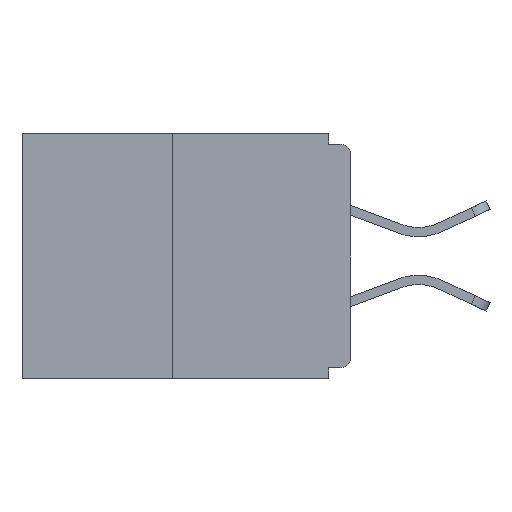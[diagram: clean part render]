
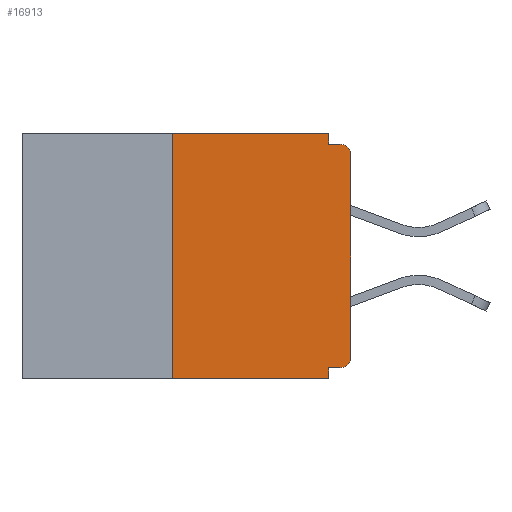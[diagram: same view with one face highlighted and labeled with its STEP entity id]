
A CAD part, left-side view. The second image highlights one B-rep face of the part: STEP entity #16913.
In plain terms, the highlighted planar face has unit normal (-1, 0, 0).
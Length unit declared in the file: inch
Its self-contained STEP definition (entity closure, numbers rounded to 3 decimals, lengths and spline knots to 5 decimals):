
#122 = EDGE_CURVE ( 'NONE', #4354, #20350, #23432, .T. ) ;
#171 = DIRECTION ( 'NONE',  ( 0., 0., -1. ) ) ;
#388 = CARTESIAN_POINT ( 'NONE',  ( 0., 0.015, -0.313 ) ) ;
#556 = ORIENTED_EDGE ( 'NONE', *, *, #22583, .T. ) ;
#1011 = ORIENTED_EDGE ( 'NONE', *, *, #21110, .F. ) ;
#1294 = ORIENTED_EDGE ( 'NONE', *, *, #122, .F. ) ;
#1313 = EDGE_CURVE ( 'NONE', #5069, #13812, #3944, .T. ) ;
#2263 = LINE ( 'NONE', #4719, #18832 ) ;
#3266 = CARTESIAN_POINT ( 'NONE',  ( 0., 0.031, 0. ) ) ;
#3462 = FACE_OUTER_BOUND ( 'NONE', #26568, .T. ) ;
#3801 = EDGE_CURVE ( 'NONE', #5069, #25397, #2263, .T. ) ;
#3944 = CIRCLE ( 'NONE', #6987, 0.015 ) ;
#4184 = EDGE_CURVE ( 'NONE', #10355, #19621, #6949, .T. ) ;
#4192 = VECTOR ( 'NONE', #171, 39.37008 ) ;
#4354 = VERTEX_POINT ( 'NONE', #3266 ) ;
#4472 = DIRECTION ( 'NONE',  ( -1., 0., 0. ) ) ;
#4643 = CARTESIAN_POINT ( 'NONE',  ( 0., 0.25, 0. ) ) ;
#4719 = CARTESIAN_POINT ( 'NONE',  ( 0., 0., -0.328 ) ) ;
#5069 = VERTEX_POINT ( 'NONE', #16992 ) ;
#5516 = DIRECTION ( 'NONE',  ( 0., 0., -1. ) ) ;
#5732 = EDGE_CURVE ( 'NONE', #25242, #19137, #12994, .T. ) ;
#6949 = LINE ( 'NONE', #4643, #9668 ) ;
#6987 = AXIS2_PLACEMENT_3D ( 'NONE', #388, #4472, #17022 ) ;
#7081 = CARTESIAN_POINT ( 'NONE',  ( 0., 0.46, 0. ) ) ;
#7282 = CARTESIAN_POINT ( 'NONE',  ( 0., 0.46, 0. ) ) ;
#7720 = VECTOR ( 'NONE', #17278, 39.37008 ) ;
#8055 = EDGE_CURVE ( 'NONE', #20350, #19137, #13653, .T. ) ;
#8170 = CARTESIAN_POINT ( 'NONE',  ( 0., 0.25, 0. ) ) ;
#8269 = ORIENTED_EDGE ( 'NONE', *, *, #3801, .F. ) ;
#8384 = VECTOR ( 'NONE', #25337, 39.37008 ) ;
#8556 = CARTESIAN_POINT ( 'NONE',  ( 0., 0.031, 0. ) ) ;
#9668 = VECTOR ( 'NONE', #25611, 39.37008 ) ;
#9705 = ORIENTED_EDGE ( 'NONE', *, *, #5732, .T. ) ;
#10355 = VERTEX_POINT ( 'NONE', #12932 ) ;
#10748 = ORIENTED_EDGE ( 'NONE', *, *, #4184, .F. ) ;
#10980 = CARTESIAN_POINT ( 'NONE',  ( 0., 0., 0. ) ) ;
#11096 = EDGE_CURVE ( 'NONE', #25397, #12016, #12307, .T. ) ;
#11197 = VECTOR ( 'NONE', #15406, 39.37008 ) ;
#11774 = PLANE ( 'NONE',  #25971 ) ;
#11776 = CARTESIAN_POINT ( 'NONE',  ( 0., 0.015, -0.015 ) ) ;
#12016 = VERTEX_POINT ( 'NONE', #12259 ) ;
#12259 = CARTESIAN_POINT ( 'NONE',  ( 0., 0.031, -0.343 ) ) ;
#12307 = LINE ( 'NONE', #25360, #4192 ) ;
#12932 = CARTESIAN_POINT ( 'NONE',  ( 0., 0.25, -0.343 ) ) ;
#12976 = CARTESIAN_POINT ( 'NONE',  ( 0., 0., -0.03 ) ) ;
#12994 = CIRCLE ( 'NONE', #13880, 0.015 ) ;
#13375 = LINE ( 'NONE', #7081, #11197 ) ;
#13478 = CARTESIAN_POINT ( 'NONE',  ( 0., 0.031, -0.015 ) ) ;
#13653 = LINE ( 'NONE', #16387, #25828 ) ;
#13812 = VERTEX_POINT ( 'NONE', #24005 ) ;
#13880 = AXIS2_PLACEMENT_3D ( 'NONE', #22102, #15992, #24150 ) ;
#14348 = CARTESIAN_POINT ( 'NONE',  ( 0., 0.46, -0.343 ) ) ;
#15406 = DIRECTION ( 'NONE',  ( 0., -1., 0. ) ) ;
#15563 = ORIENTED_EDGE ( 'NONE', *, *, #17187, .T. ) ;
#15743 = DIRECTION ( 'NONE',  ( 1., 0., 0. ) ) ;
#15992 = DIRECTION ( 'NONE',  ( -1., 0., 0. ) ) ;
#16387 = CARTESIAN_POINT ( 'NONE',  ( 0., 0., -0.015 ) ) ;
#16913 = ADVANCED_FACE ( 'NONE', ( #3462 ), #11774, .F. ) ;
#16992 = CARTESIAN_POINT ( 'NONE',  ( 0., 0.015, -0.328 ) ) ;
#17022 = DIRECTION ( 'NONE',  ( 0., 0., -1. ) ) ;
#17187 = EDGE_CURVE ( 'NONE', #13812, #25242, #21492, .T. ) ;
#17278 = DIRECTION ( 'NONE',  ( 0., 0., 1. ) ) ;
#18832 = VECTOR ( 'NONE', #23376, 39.37008 ) ;
#19029 = ORIENTED_EDGE ( 'NONE', *, *, #11096, .F. ) ;
#19137 = VERTEX_POINT ( 'NONE', #11776 ) ;
#19621 = VERTEX_POINT ( 'NONE', #8170 ) ;
#19953 = CARTESIAN_POINT ( 'NONE',  ( 0., 0.031, -0.328 ) ) ;
#20350 = VERTEX_POINT ( 'NONE', #13478 ) ;
#20475 = DIRECTION ( 'NONE',  ( 0., -1., 0. ) ) ;
#21110 = EDGE_CURVE ( 'NONE', #19621, #4354, #13375, .T. ) ;
#21492 = LINE ( 'NONE', #10980, #7720 ) ;
#22102 = CARTESIAN_POINT ( 'NONE',  ( 0., 0.015, -0.03 ) ) ;
#22583 = EDGE_CURVE ( 'NONE', #10355, #12016, #24291, .T. ) ;
#22651 = DIRECTION ( 'NONE',  ( 0., -1., 0. ) ) ;
#23376 = DIRECTION ( 'NONE',  ( 0., 1., 0. ) ) ;
#23432 = LINE ( 'NONE', #8556, #8384 ) ;
#24005 = CARTESIAN_POINT ( 'NONE',  ( 0., 0., -0.313 ) ) ;
#24150 = DIRECTION ( 'NONE',  ( 0., 0., -1. ) ) ;
#24291 = LINE ( 'NONE', #14348, #24751 ) ;
#24751 = VECTOR ( 'NONE', #22651, 39.37008 ) ;
#25049 = ORIENTED_EDGE ( 'NONE', *, *, #1313, .T. ) ;
#25242 = VERTEX_POINT ( 'NONE', #12976 ) ;
#25337 = DIRECTION ( 'NONE',  ( 0., 0., -1. ) ) ;
#25360 = CARTESIAN_POINT ( 'NONE',  ( 0., 0.031, -0.343 ) ) ;
#25397 = VERTEX_POINT ( 'NONE', #19953 ) ;
#25611 = DIRECTION ( 'NONE',  ( 0., 0., 1. ) ) ;
#25828 = VECTOR ( 'NONE', #20475, 39.37008 ) ;
#25971 = AXIS2_PLACEMENT_3D ( 'NONE', #7282, #15743, #5516 ) ;
#26568 = EDGE_LOOP ( 'NONE', ( #1011, #10748, #556, #19029, #8269, #25049, #15563, #9705, #26643, #1294 ) ) ;
#26643 = ORIENTED_EDGE ( 'NONE', *, *, #8055, .F. ) ;
